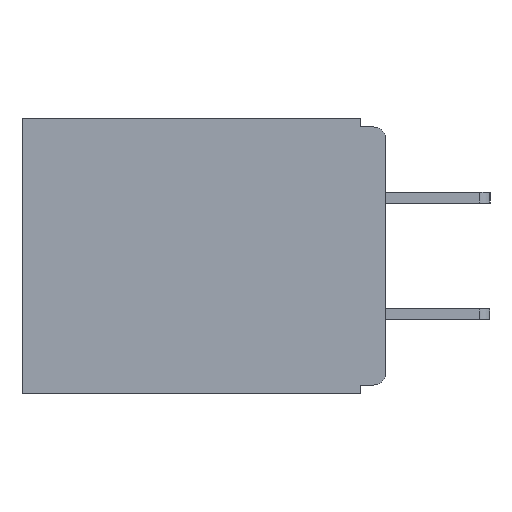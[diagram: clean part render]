
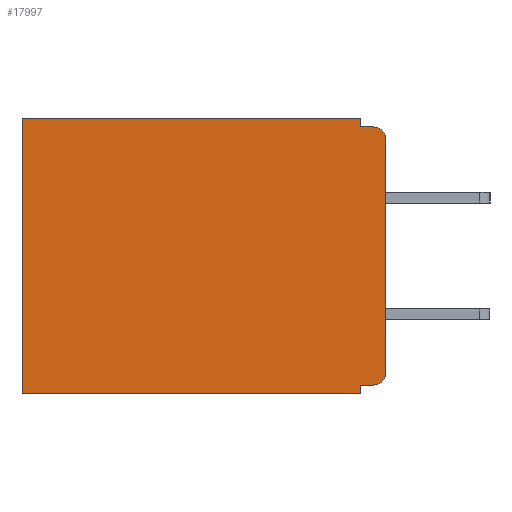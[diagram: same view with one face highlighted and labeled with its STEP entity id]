
A CAD part, left-side view. The second image highlights one B-rep face of the part: STEP entity #17997.
In plain terms, the highlighted planar face has unit normal (-1, 0, 0).
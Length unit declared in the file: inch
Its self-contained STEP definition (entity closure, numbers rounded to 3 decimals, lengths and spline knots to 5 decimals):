
#573 = DIRECTION ( 'NONE',  ( 0., 0., -1. ) ) ;
#972 = CARTESIAN_POINT ( 'NONE',  ( 0.3, 0.031, -0.33 ) ) ;
#1111 = LINE ( 'NONE', #17551, #11146 ) ;
#1362 = VECTOR ( 'NONE', #9953, 39.37008 ) ;
#1368 = DIRECTION ( 'NONE',  ( -1., 0., 0. ) ) ;
#2201 = CARTESIAN_POINT ( 'NONE',  ( 0.3, 0.015, -0.01 ) ) ;
#2403 = LINE ( 'NONE', #12667, #7100 ) ;
#2554 = CARTESIAN_POINT ( 'NONE',  ( 0.3, 0.437, 0. ) ) ;
#2837 = VERTEX_POINT ( 'NONE', #4824 ) ;
#3304 = ORIENTED_EDGE ( 'NONE', *, *, #15334, .T. ) ;
#3683 = DIRECTION ( 'NONE',  ( 0., 0., -1. ) ) ;
#3717 = EDGE_CURVE ( 'NONE', #2837, #9524, #22246, .T. ) ;
#3927 = CARTESIAN_POINT ( 'NONE',  ( 0.3, 0.031, -0.01 ) ) ;
#4004 = DIRECTION ( 'NONE',  ( 0., -1., 0. ) ) ;
#4248 = DIRECTION ( 'NONE',  ( -1., 0., 0. ) ) ;
#4260 = ORIENTED_EDGE ( 'NONE', *, *, #24695, .F. ) ;
#4616 = DIRECTION ( 'NONE',  ( 0., 0., -1. ) ) ;
#4824 = CARTESIAN_POINT ( 'NONE',  ( 0.3, 0.031, 0. ) ) ;
#4888 = ORIENTED_EDGE ( 'NONE', *, *, #3717, .T. ) ;
#5500 = EDGE_LOOP ( 'NONE', ( #20488, #16506, #14305, #4260, #4888, #21383, #6133, #12104, #23834, #3304 ) ) ;
#5513 = LINE ( 'NONE', #8751, #16181 ) ;
#5600 = VERTEX_POINT ( 'NONE', #6003 ) ;
#6003 = CARTESIAN_POINT ( 'NONE',  ( 0.3, 0.031, -0.33 ) ) ;
#6133 = ORIENTED_EDGE ( 'NONE', *, *, #6920, .F. ) ;
#6920 = EDGE_CURVE ( 'NONE', #5600, #11378, #9064, .T. ) ;
#7100 = VECTOR ( 'NONE', #4616, 39.37008 ) ;
#7993 = CARTESIAN_POINT ( 'NONE',  ( 0.3, 0., -0.33 ) ) ;
#8080 = DIRECTION ( 'NONE',  ( 0., 1., 0. ) ) ;
#8116 = EDGE_CURVE ( 'NONE', #22360, #23751, #8986, .T. ) ;
#8130 = VERTEX_POINT ( 'NONE', #12081 ) ;
#8262 = AXIS2_PLACEMENT_3D ( 'NONE', #16254, #4248, #18234 ) ;
#8751 = CARTESIAN_POINT ( 'NONE',  ( 0.3, 0., -0.32 ) ) ;
#8986 = LINE ( 'NONE', #18007, #23519 ) ;
#9064 = LINE ( 'NONE', #7993, #24841 ) ;
#9140 = DIRECTION ( 'NONE',  ( 0., 0., -1. ) ) ;
#9290 = EDGE_CURVE ( 'NONE', #9524, #11378, #17972, .T. ) ;
#9524 = VERTEX_POINT ( 'NONE', #2554 ) ;
#9857 = LINE ( 'NONE', #972, #19822 ) ;
#9953 = DIRECTION ( 'NONE',  ( 0., 0., -1. ) ) ;
#10323 = AXIS2_PLACEMENT_3D ( 'NONE', #14523, #12568, #573 ) ;
#11146 = VECTOR ( 'NONE', #3683, 39.37008 ) ;
#11378 = VERTEX_POINT ( 'NONE', #18851 ) ;
#11850 = CIRCLE ( 'NONE', #13586, 0.015 ) ;
#12081 = CARTESIAN_POINT ( 'NONE',  ( 0.3, 0.015, -0.32 ) ) ;
#12104 = ORIENTED_EDGE ( 'NONE', *, *, #22048, .F. ) ;
#12415 = VERTEX_POINT ( 'NONE', #16041 ) ;
#12568 = DIRECTION ( 'NONE',  ( 1., 0., 0. ) ) ;
#12667 = CARTESIAN_POINT ( 'NONE',  ( 0.3, 0., -0.33 ) ) ;
#13388 = CARTESIAN_POINT ( 'NONE',  ( 0.3, 0.015, -0.305 ) ) ;
#13586 = AXIS2_PLACEMENT_3D ( 'NONE', #13388, #1368, #15408 ) ;
#13686 = VERTEX_POINT ( 'NONE', #21655 ) ;
#13885 = CARTESIAN_POINT ( 'NONE',  ( 0.3, 0.437, -0.33 ) ) ;
#14305 = ORIENTED_EDGE ( 'NONE', *, *, #8116, .F. ) ;
#14523 = CARTESIAN_POINT ( 'NONE',  ( 0.3, 0., -0.33 ) ) ;
#14720 = CARTESIAN_POINT ( 'NONE',  ( 0.3, 0., -0.025 ) ) ;
#15334 = EDGE_CURVE ( 'NONE', #8130, #12415, #11850, .T. ) ;
#15408 = DIRECTION ( 'NONE',  ( 0., 0., -1. ) ) ;
#16041 = CARTESIAN_POINT ( 'NONE',  ( 0.3, 0., -0.305 ) ) ;
#16176 = EDGE_CURVE ( 'NONE', #24518, #12415, #2403, .T. ) ;
#16181 = VECTOR ( 'NONE', #20671, 39.37008 ) ;
#16254 = CARTESIAN_POINT ( 'NONE',  ( 0.3, 0.015, -0.025 ) ) ;
#16506 = ORIENTED_EDGE ( 'NONE', *, *, #20619, .T. ) ;
#16778 = FACE_OUTER_BOUND ( 'NONE', #5500, .T. ) ;
#17086 = VECTOR ( 'NONE', #24664, 39.37008 ) ;
#17551 = CARTESIAN_POINT ( 'NONE',  ( 0.3, 0.031, 0. ) ) ;
#17972 = LINE ( 'NONE', #13885, #1362 ) ;
#17997 = ADVANCED_FACE ( 'NONE', ( #16778 ), #24405, .F. ) ;
#18007 = CARTESIAN_POINT ( 'NONE',  ( 0.3, 0., -0.01 ) ) ;
#18234 = DIRECTION ( 'NONE',  ( 0., 0., -1. ) ) ;
#18851 = CARTESIAN_POINT ( 'NONE',  ( 0.3, 0.437, -0.33 ) ) ;
#19822 = VECTOR ( 'NONE', #9140, 39.37008 ) ;
#19908 = CIRCLE ( 'NONE', #8262, 0.015 ) ;
#20488 = ORIENTED_EDGE ( 'NONE', *, *, #16176, .F. ) ;
#20619 = EDGE_CURVE ( 'NONE', #24518, #23751, #19908, .T. ) ;
#20671 = DIRECTION ( 'NONE',  ( 0., 1., 0. ) ) ;
#21383 = ORIENTED_EDGE ( 'NONE', *, *, #9290, .T. ) ;
#21655 = CARTESIAN_POINT ( 'NONE',  ( 0.3, 0.031, -0.32 ) ) ;
#22048 = EDGE_CURVE ( 'NONE', #13686, #5600, #9857, .T. ) ;
#22246 = LINE ( 'NONE', #24213, #17086 ) ;
#22360 = VERTEX_POINT ( 'NONE', #3927 ) ;
#23519 = VECTOR ( 'NONE', #4004, 39.37008 ) ;
#23751 = VERTEX_POINT ( 'NONE', #2201 ) ;
#23834 = ORIENTED_EDGE ( 'NONE', *, *, #24540, .F. ) ;
#24213 = CARTESIAN_POINT ( 'NONE',  ( 0.3, 0., 0. ) ) ;
#24405 = PLANE ( 'NONE',  #10323 ) ;
#24518 = VERTEX_POINT ( 'NONE', #14720 ) ;
#24540 = EDGE_CURVE ( 'NONE', #8130, #13686, #5513, .T. ) ;
#24664 = DIRECTION ( 'NONE',  ( 0., 1., 0. ) ) ;
#24695 = EDGE_CURVE ( 'NONE', #2837, #22360, #1111, .T. ) ;
#24841 = VECTOR ( 'NONE', #8080, 39.37008 ) ;
